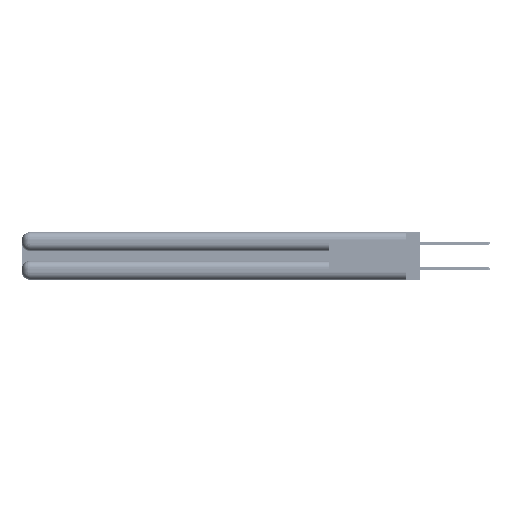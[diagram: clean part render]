
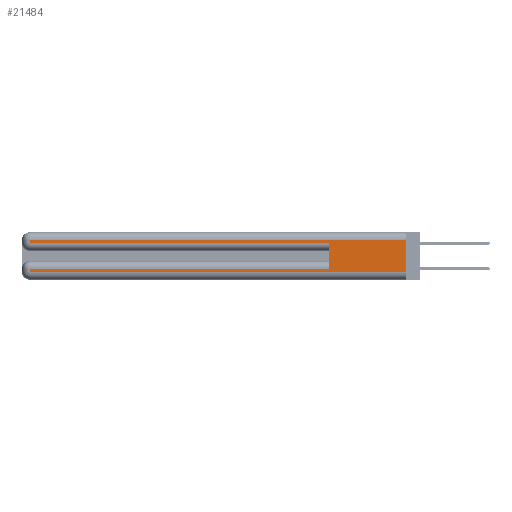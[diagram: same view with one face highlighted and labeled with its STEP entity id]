
A CAD part, left-side view. The second image highlights one B-rep face of the part: STEP entity #21484.
In plain terms, the highlighted planar face has unit normal (-1, 0, 0).
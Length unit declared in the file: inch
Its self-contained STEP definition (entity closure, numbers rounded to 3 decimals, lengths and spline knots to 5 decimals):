
#1312 = CARTESIAN_POINT ( 'NONE',  ( 0., 2.94, 0.31 ) ) ;
#1839 = CARTESIAN_POINT ( 'NONE',  ( 0., 0., 0.06 ) ) ;
#1978 = DIRECTION ( 'NONE',  ( 0., 0., -1. ) ) ;
#2130 = LINE ( 'NONE', #47871, #23448 ) ;
#2171 = VERTEX_POINT ( 'NONE', #1839 ) ;
#2504 = VECTOR ( 'NONE', #8536, 39.37008 ) ;
#3642 = ORIENTED_EDGE ( 'NONE', *, *, #16282, .F. ) ;
#5547 = EDGE_CURVE ( 'NONE', #18170, #23319, #46224, .T. ) ;
#6366 = DIRECTION ( 'NONE',  ( 0., 0., 1. ) ) ;
#6677 = ORIENTED_EDGE ( 'NONE', *, *, #53696, .T. ) ;
#8536 = DIRECTION ( 'NONE',  ( 0., 0., -1. ) ) ;
#11875 = VECTOR ( 'NONE', #32891, 39.37008 ) ;
#12892 = CARTESIAN_POINT ( 'NONE',  ( 0., 2.94, 0.37 ) ) ;
#15147 = ORIENTED_EDGE ( 'NONE', *, *, #49277, .T. ) ;
#15779 = DIRECTION ( 'NONE',  ( 0., 0., -1. ) ) ;
#15842 = VERTEX_POINT ( 'NONE', #1312 ) ;
#15983 = CARTESIAN_POINT ( 'NONE',  ( 0., 0., 0.085 ) ) ;
#16282 = EDGE_CURVE ( 'NONE', #31262, #2171, #25103, .T. ) ;
#16379 = AXIS2_PLACEMENT_3D ( 'NONE', #39698, #27419, #1978 ) ;
#16762 = VERTEX_POINT ( 'NONE', #53496 ) ;
#16777 = EDGE_CURVE ( 'NONE', #18170, #46749, #23191, .T. ) ;
#18170 = VERTEX_POINT ( 'NONE', #39006 ) ;
#18360 = CARTESIAN_POINT ( 'NONE',  ( 0., 0., 0.06 ) ) ;
#18964 = PLANE ( 'NONE',  #16379 ) ;
#20479 = LINE ( 'NONE', #12892, #29025 ) ;
#21484 = ADVANCED_FACE ( 'NONE', ( #30809 ), #18964, .F. ) ;
#22015 = ORIENTED_EDGE ( 'NONE', *, *, #16777, .T. ) ;
#23026 = CARTESIAN_POINT ( 'NONE',  ( 0., 0.6, 0.285 ) ) ;
#23191 = LINE ( 'NONE', #15983, #11875 ) ;
#23319 = VERTEX_POINT ( 'NONE', #23026 ) ;
#23448 = VECTOR ( 'NONE', #52101, 39.37008 ) ;
#23486 = ORIENTED_EDGE ( 'NONE', *, *, #47929, .T. ) ;
#24097 = CARTESIAN_POINT ( 'NONE',  ( 0., 0., 0.31 ) ) ;
#25103 = LINE ( 'NONE', #42267, #2504 ) ;
#26965 = EDGE_LOOP ( 'NONE', ( #3642, #51159, #23486, #48240, #45642, #22015, #6677, #15147 ) ) ;
#27316 = LINE ( 'NONE', #48394, #38471 ) ;
#27419 = DIRECTION ( 'NONE',  ( 1., 0., 0. ) ) ;
#27553 = LINE ( 'NONE', #40934, #48435 ) ;
#29025 = VECTOR ( 'NONE', #37961, 39.37008 ) ;
#30809 = FACE_OUTER_BOUND ( 'NONE', #26965, .T. ) ;
#31262 = VERTEX_POINT ( 'NONE', #24097 ) ;
#31741 = CARTESIAN_POINT ( 'NONE',  ( 0., 0.6, 0.145 ) ) ;
#32891 = DIRECTION ( 'NONE',  ( 0., 1., 0. ) ) ;
#33733 = CARTESIAN_POINT ( 'NONE',  ( 0., 2.94, 0.085 ) ) ;
#35381 = CARTESIAN_POINT ( 'NONE',  ( 0., 2.94, 0.285 ) ) ;
#37961 = DIRECTION ( 'NONE',  ( 0., 0., -1. ) ) ;
#38324 = EDGE_CURVE ( 'NONE', #39237, #23319, #27316, .T. ) ;
#38471 = VECTOR ( 'NONE', #52618, 39.37008 ) ;
#39006 = CARTESIAN_POINT ( 'NONE',  ( 0., 0.6, 0.085 ) ) ;
#39097 = VECTOR ( 'NONE', #6366, 39.37008 ) ;
#39237 = VERTEX_POINT ( 'NONE', #35381 ) ;
#39698 = CARTESIAN_POINT ( 'NONE',  ( 0., 0., 0.37 ) ) ;
#40934 = CARTESIAN_POINT ( 'NONE',  ( 0., 2.94, 0.37 ) ) ;
#42267 = CARTESIAN_POINT ( 'NONE',  ( 0., 0., 0.37 ) ) ;
#43468 = DIRECTION ( 'NONE',  ( 0., -1., 0. ) ) ;
#45155 = EDGE_CURVE ( 'NONE', #31262, #15842, #2130, .T. ) ;
#45642 = ORIENTED_EDGE ( 'NONE', *, *, #5547, .F. ) ;
#45882 = LINE ( 'NONE', #18360, #47168 ) ;
#46224 = LINE ( 'NONE', #31741, #39097 ) ;
#46749 = VERTEX_POINT ( 'NONE', #33733 ) ;
#47168 = VECTOR ( 'NONE', #43468, 39.37008 ) ;
#47871 = CARTESIAN_POINT ( 'NONE',  ( 0., 0., 0.31 ) ) ;
#47929 = EDGE_CURVE ( 'NONE', #15842, #39237, #20479, .T. ) ;
#48240 = ORIENTED_EDGE ( 'NONE', *, *, #38324, .T. ) ;
#48394 = CARTESIAN_POINT ( 'NONE',  ( 0., 0., 0.285 ) ) ;
#48435 = VECTOR ( 'NONE', #15779, 39.37008 ) ;
#49277 = EDGE_CURVE ( 'NONE', #16762, #2171, #45882, .T. ) ;
#51159 = ORIENTED_EDGE ( 'NONE', *, *, #45155, .T. ) ;
#52101 = DIRECTION ( 'NONE',  ( 0., 1., 0. ) ) ;
#52618 = DIRECTION ( 'NONE',  ( 0., -1., 0. ) ) ;
#53496 = CARTESIAN_POINT ( 'NONE',  ( 0., 2.94, 0.06 ) ) ;
#53696 = EDGE_CURVE ( 'NONE', #46749, #16762, #27553, .T. ) ;
